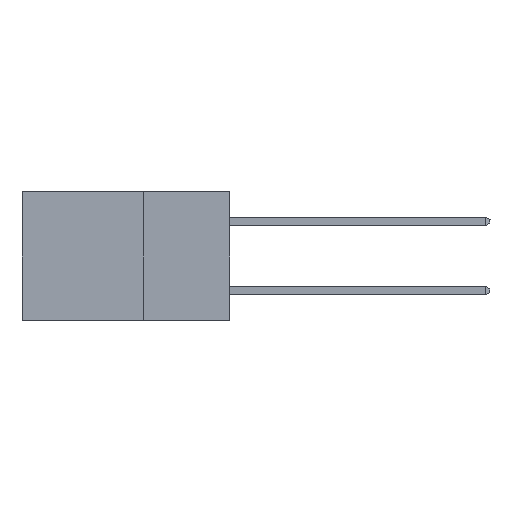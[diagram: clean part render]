
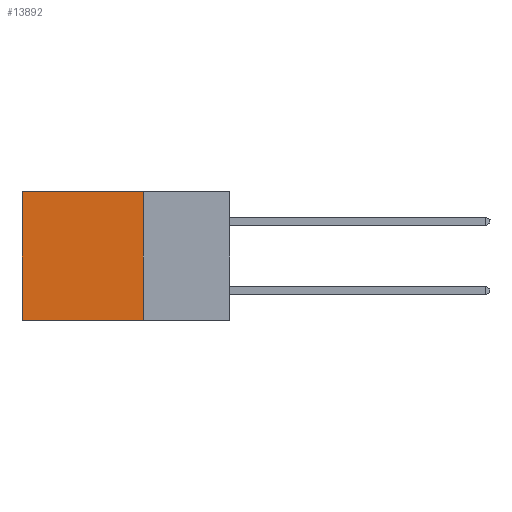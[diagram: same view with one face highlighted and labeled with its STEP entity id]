
A CAD part, left-side view. The second image highlights one B-rep face of the part: STEP entity #13892.
In plain terms, the highlighted planar face has unit normal (-1, 0, 0).
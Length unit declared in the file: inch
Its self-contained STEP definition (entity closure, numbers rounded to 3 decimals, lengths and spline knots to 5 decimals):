
#108 = VECTOR ( 'NONE', #11260, 39.37008 ) ;
#753 = CARTESIAN_POINT ( 'NONE',  ( 0.2615, 0.25, -0.37 ) ) ;
#969 = LINE ( 'NONE', #9055, #9304 ) ;
#1118 = LINE ( 'NONE', #10313, #7123 ) ;
#1160 = DIRECTION ( 'NONE',  ( 0., 1., 0. ) ) ;
#1161 = CARTESIAN_POINT ( 'NONE',  ( 0.2615, 0.6, -0.37 ) ) ;
#1333 = DIRECTION ( 'NONE',  ( 1., 0., 0. ) ) ;
#1555 = ORIENTED_EDGE ( 'NONE', *, *, #14419, .T. ) ;
#2200 = CARTESIAN_POINT ( 'NONE',  ( 0.2615, 0.6, 0. ) ) ;
#2689 = EDGE_CURVE ( 'NONE', #6832, #12866, #13948, .T. ) ;
#3265 = AXIS2_PLACEMENT_3D ( 'NONE', #9332, #1333, #6008 ) ;
#4541 = DIRECTION ( 'NONE',  ( 0., 0., -1. ) ) ;
#4595 = FACE_OUTER_BOUND ( 'NONE', #6065, .T. ) ;
#5603 = LINE ( 'NONE', #753, #108 ) ;
#5724 = DIRECTION ( 'NONE',  ( 0., 1., 0. ) ) ;
#5748 = ORIENTED_EDGE ( 'NONE', *, *, #12726, .F. ) ;
#6008 = DIRECTION ( 'NONE',  ( 0., 0., -1. ) ) ;
#6065 = EDGE_LOOP ( 'NONE', ( #1555, #7105, #5748, #6813 ) ) ;
#6813 = ORIENTED_EDGE ( 'NONE', *, *, #2689, .T. ) ;
#6832 = VERTEX_POINT ( 'NONE', #11505 ) ;
#7105 = ORIENTED_EDGE ( 'NONE', *, *, #13887, .F. ) ;
#7123 = VECTOR ( 'NONE', #5724, 39.37008 ) ;
#8931 = VECTOR ( 'NONE', #1160, 39.37008 ) ;
#9055 = CARTESIAN_POINT ( 'NONE',  ( 0.2615, 0.6, -0.37 ) ) ;
#9304 = VECTOR ( 'NONE', #4541, 39.37008 ) ;
#9332 = CARTESIAN_POINT ( 'NONE',  ( 0.2615, 0.25, -0.37 ) ) ;
#10313 = CARTESIAN_POINT ( 'NONE',  ( 0.2615, 0.25, -0.37 ) ) ;
#10594 = PLANE ( 'NONE',  #3265 ) ;
#11102 = VERTEX_POINT ( 'NONE', #1161 ) ;
#11260 = DIRECTION ( 'NONE',  ( 0., 0., -1. ) ) ;
#11505 = CARTESIAN_POINT ( 'NONE',  ( 0.2615, 0.25, 0. ) ) ;
#12726 = EDGE_CURVE ( 'NONE', #6832, #12920, #5603, .T. ) ;
#12813 = CARTESIAN_POINT ( 'NONE',  ( 0.2615, 0.25, -0.37 ) ) ;
#12866 = VERTEX_POINT ( 'NONE', #2200 ) ;
#12920 = VERTEX_POINT ( 'NONE', #12813 ) ;
#13887 = EDGE_CURVE ( 'NONE', #12920, #11102, #1118, .T. ) ;
#13892 = ADVANCED_FACE ( 'NONE', ( #4595 ), #10594, .F. ) ;
#13948 = LINE ( 'NONE', #14025, #8931 ) ;
#14025 = CARTESIAN_POINT ( 'NONE',  ( 0.2615, 0.25, 0. ) ) ;
#14419 = EDGE_CURVE ( 'NONE', #12866, #11102, #969, .T. ) ;
